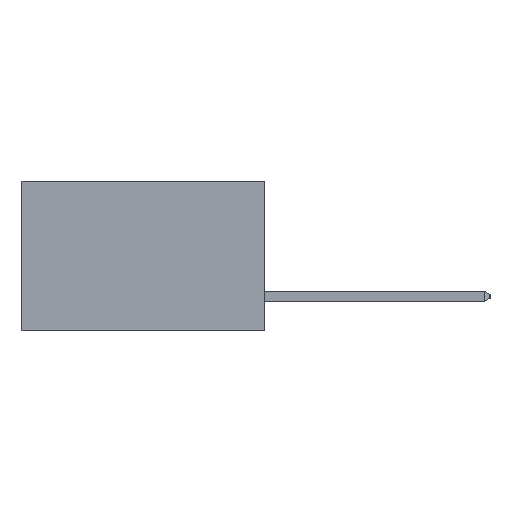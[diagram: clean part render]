
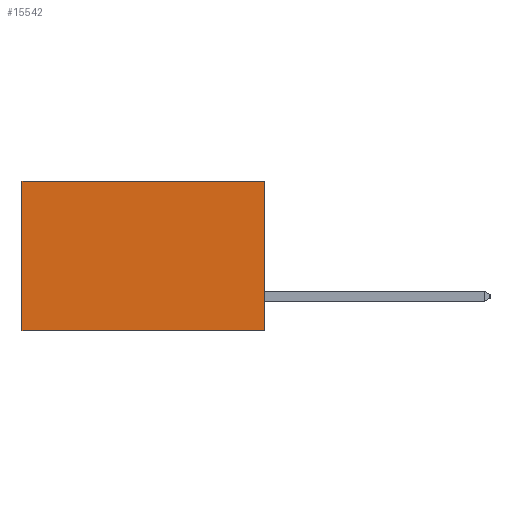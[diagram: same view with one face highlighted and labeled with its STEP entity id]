
A CAD part, left-side view. The second image highlights one B-rep face of the part: STEP entity #15542.
In plain terms, the highlighted planar face has unit normal (-1, 0, 0).
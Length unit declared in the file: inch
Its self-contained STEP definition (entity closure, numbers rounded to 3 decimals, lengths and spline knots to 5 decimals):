
#267 = VECTOR ( 'NONE', #16859, 39.37008 ) ;
#744 = LINE ( 'NONE', #18280, #5588 ) ;
#1136 = VERTEX_POINT ( 'NONE', #20044 ) ;
#2129 = EDGE_CURVE ( 'NONE', #1136, #3231, #10570, .T. ) ;
#2960 = VERTEX_POINT ( 'NONE', #12202 ) ;
#3231 = VERTEX_POINT ( 'NONE', #8223 ) ;
#3938 = DIRECTION ( 'NONE',  ( 0., 0., -1. ) ) ;
#5588 = VECTOR ( 'NONE', #20268, 39.37008 ) ;
#5760 = CARTESIAN_POINT ( 'NONE',  ( 0.2615, 0., 0. ) ) ;
#6234 = EDGE_CURVE ( 'NONE', #2960, #3231, #19742, .T. ) ;
#6848 = AXIS2_PLACEMENT_3D ( 'NONE', #25697, #16078, #3938 ) ;
#7565 = EDGE_LOOP ( 'NONE', ( #15232, #10562, #16646, #10323 ) ) ;
#7796 = DIRECTION ( 'NONE',  ( 0., 1., 0. ) ) ;
#8223 = CARTESIAN_POINT ( 'NONE',  ( 0.2615, 0.6, -0.37 ) ) ;
#10075 = DIRECTION ( 'NONE',  ( 0., 0., -1. ) ) ;
#10323 = ORIENTED_EDGE ( 'NONE', *, *, #16675, .T. ) ;
#10526 = CARTESIAN_POINT ( 'NONE',  ( 0.2615, 0.6, -0.37 ) ) ;
#10562 = ORIENTED_EDGE ( 'NONE', *, *, #2129, .F. ) ;
#10570 = LINE ( 'NONE', #16352, #267 ) ;
#12202 = CARTESIAN_POINT ( 'NONE',  ( 0.2615, 0.6, 0. ) ) ;
#12809 = FACE_OUTER_BOUND ( 'NONE', #7565, .T. ) ;
#15232 = ORIENTED_EDGE ( 'NONE', *, *, #6234, .T. ) ;
#15542 = ADVANCED_FACE ( 'NONE', ( #12809 ), #21887, .F. ) ;
#16078 = DIRECTION ( 'NONE',  ( 1., 0., 0. ) ) ;
#16352 = CARTESIAN_POINT ( 'NONE',  ( 0.2615, 0., -0.37 ) ) ;
#16646 = ORIENTED_EDGE ( 'NONE', *, *, #19468, .F. ) ;
#16675 = EDGE_CURVE ( 'NONE', #20164, #2960, #21672, .T. ) ;
#16859 = DIRECTION ( 'NONE',  ( 0., 1., 0. ) ) ;
#17091 = VECTOR ( 'NONE', #7796, 39.37008 ) ;
#18280 = CARTESIAN_POINT ( 'NONE',  ( 0.2615, 0., -0.37 ) ) ;
#19468 = EDGE_CURVE ( 'NONE', #20164, #1136, #744, .T. ) ;
#19742 = LINE ( 'NONE', #10526, #24773 ) ;
#20044 = CARTESIAN_POINT ( 'NONE',  ( 0.2615, 0., -0.37 ) ) ;
#20164 = VERTEX_POINT ( 'NONE', #23783 ) ;
#20268 = DIRECTION ( 'NONE',  ( 0., 0., -1. ) ) ;
#21672 = LINE ( 'NONE', #5760, #17091 ) ;
#21887 = PLANE ( 'NONE',  #6848 ) ;
#23783 = CARTESIAN_POINT ( 'NONE',  ( 0.2615, 0., 0. ) ) ;
#24773 = VECTOR ( 'NONE', #10075, 39.37008 ) ;
#25697 = CARTESIAN_POINT ( 'NONE',  ( 0.2615, 0., -0.37 ) ) ;
